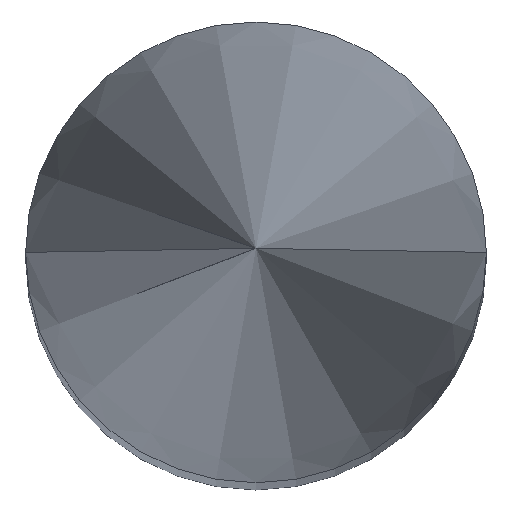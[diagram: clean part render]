
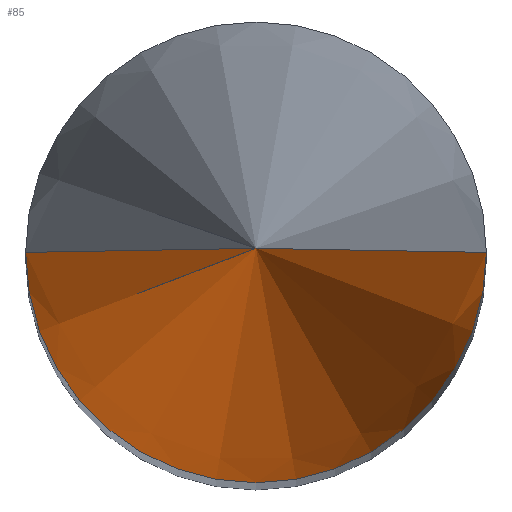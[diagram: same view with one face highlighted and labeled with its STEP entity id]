
A CAD part, top view. The second image highlights one B-rep face of the part: STEP entity #85.
In plain terms, the highlighted conical face has half-angle 5.711 degrees and reference radius 0.5 mm.
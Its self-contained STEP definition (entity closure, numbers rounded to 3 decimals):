
#3 = CARTESIAN_POINT ( 'NONE',  ( 0.5, 0., 9. ) ) ;
#6 = ORIENTED_EDGE ( 'NONE', *, *, #153, .T. ) ;
#7 = EDGE_LOOP ( 'NONE', ( #82, #6, #30 ) ) ;
#11 = FACE_OUTER_BOUND ( 'NONE', #7, .T. ) ;
#13 = CARTESIAN_POINT ( 'NONE',  ( 0.5, 0., 9. ) ) ;
#24 = CIRCLE ( 'NONE', #46, 0.5 ) ;
#27 = DIRECTION ( 'NONE',  ( 0., 0., -1. ) ) ;
#29 = VERTEX_POINT ( 'NONE', #128 ) ;
#30 = ORIENTED_EDGE ( 'NONE', *, *, #145, .F. ) ;
#46 = AXIS2_PLACEMENT_3D ( 'NONE', #158, #118, #95 ) ;
#49 = LINE ( 'NONE', #161, #52 ) ;
#52 = VECTOR ( 'NONE', #117, 1000. ) ;
#58 = CONICAL_SURFACE ( 'NONE', #133, 0.5, 0.1 ) ;
#63 = VECTOR ( 'NONE', #114, 1000. ) ;
#68 = LINE ( 'NONE', #13, #63 ) ;
#82 = ORIENTED_EDGE ( 'NONE', *, *, #146, .F. ) ;
#85 = ADVANCED_FACE ( 'NONE', ( #11 ), #58, .T. ) ;
#95 = DIRECTION ( 'NONE',  ( 1., 0., 0. ) ) ;
#96 = VERTEX_POINT ( 'NONE', #100 ) ;
#100 = CARTESIAN_POINT ( 'NONE',  ( -0.5, 0., 9. ) ) ;
#101 = VERTEX_POINT ( 'NONE', #3 ) ;
#107 = CARTESIAN_POINT ( 'NONE',  ( 0., 0., 9. ) ) ;
#114 = DIRECTION ( 'NONE',  ( 0.1, 0., -0.995 ) ) ;
#117 = DIRECTION ( 'NONE',  ( -0.1, 0., -0.995 ) ) ;
#118 = DIRECTION ( 'NONE',  ( 0., 0., -1. ) ) ;
#127 = DIRECTION ( 'NONE',  ( -1., 0., 0. ) ) ;
#128 = CARTESIAN_POINT ( 'NONE',  ( 0., 0., 14. ) ) ;
#133 = AXIS2_PLACEMENT_3D ( 'NONE', #107, #27, #127 ) ;
#145 = EDGE_CURVE ( 'NONE', #101, #96, #24, .T. ) ;
#146 = EDGE_CURVE ( 'NONE', #29, #101, #68, .T. ) ;
#153 = EDGE_CURVE ( 'NONE', #29, #96, #49, .T. ) ;
#158 = CARTESIAN_POINT ( 'NONE',  ( 0., 0., 9. ) ) ;
#161 = CARTESIAN_POINT ( 'NONE',  ( -0.5, 0., 9. ) ) ;
